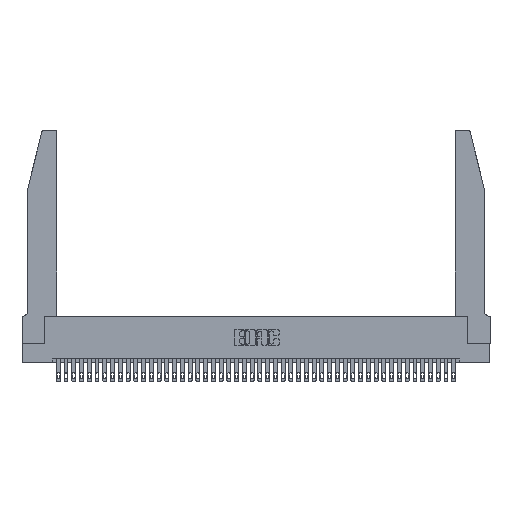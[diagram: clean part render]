
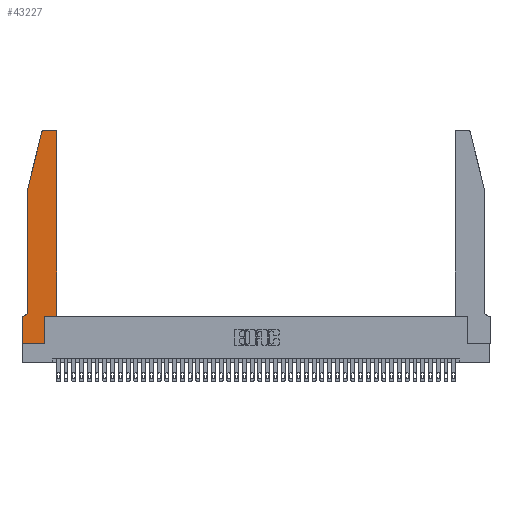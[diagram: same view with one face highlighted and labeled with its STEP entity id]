
A CAD part, top view. The second image highlights one B-rep face of the part: STEP entity #43227.
In plain terms, the highlighted planar face has unit normal (0, 0, 1).
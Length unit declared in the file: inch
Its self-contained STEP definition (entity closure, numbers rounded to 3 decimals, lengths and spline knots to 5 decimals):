
#622 = DIRECTION ( 'NONE',  ( 1., 0., 0. ) ) ;
#659 = CARTESIAN_POINT ( 'NONE',  ( 0.0755, 2., 0.37 ) ) ;
#669 = VECTOR ( 'NONE', #16665, 39.37008 ) ;
#737 = EDGE_CURVE ( 'NONE', #5990, #23715, #5614, .T. ) ;
#746 = CARTESIAN_POINT ( 'NONE',  ( 0., 0., 0.37 ) ) ;
#941 = ORIENTED_EDGE ( 'NONE', *, *, #5245, .T. ) ;
#997 = AXIS2_PLACEMENT_3D ( 'NONE', #36835, #16348, #6878 ) ;
#1511 = VECTOR ( 'NONE', #34102, 39.37008 ) ;
#1585 = CARTESIAN_POINT ( 'NONE',  ( 0.0755, 2., 0.37 ) ) ;
#1917 = CARTESIAN_POINT ( 'NONE',  ( 0.4205, 2.72, 0.37 ) ) ;
#2085 = ORIENTED_EDGE ( 'NONE', *, *, #23469, .T. ) ;
#2121 = CARTESIAN_POINT ( 'NONE',  ( 0.0055, 0.35, 0.37 ) ) ;
#2169 = CARTESIAN_POINT ( 'NONE',  ( 0.0755, 0.42, 0.37 ) ) ;
#2500 = VERTEX_POINT ( 'NONE', #10021 ) ;
#2548 = VECTOR ( 'NONE', #10915, 39.37008 ) ;
#2983 = ORIENTED_EDGE ( 'NONE', *, *, #7462, .T. ) ;
#3103 = LINE ( 'NONE', #7789, #33098 ) ;
#4253 = VERTEX_POINT ( 'NONE', #24891 ) ;
#4413 = VERTEX_POINT ( 'NONE', #15961 ) ;
#5015 = ORIENTED_EDGE ( 'NONE', *, *, #9977, .T. ) ;
#5245 = EDGE_CURVE ( 'NONE', #37400, #27369, #27476, .T. ) ;
#5614 = LINE ( 'NONE', #23602, #23258 ) ;
#5781 = VECTOR ( 'NONE', #25886, 39.37008 ) ;
#5990 = VERTEX_POINT ( 'NONE', #17314 ) ;
#6348 = DIRECTION ( 'NONE',  ( 0., -1., 0. ) ) ;
#6668 = EDGE_CURVE ( 'NONE', #4413, #11718, #29048, .T. ) ;
#6878 = DIRECTION ( 'NONE',  ( 1., 0., 0. ) ) ;
#6927 = EDGE_CURVE ( 'NONE', #13416, #5990, #22099, .T. ) ;
#7017 = LINE ( 'NONE', #14941, #35959 ) ;
#7110 = VECTOR ( 'NONE', #24988, 39.37008 ) ;
#7462 = EDGE_CURVE ( 'NONE', #28771, #40537, #7017, .T. ) ;
#7734 = ORIENTED_EDGE ( 'NONE', *, *, #6668, .T. ) ;
#7789 = CARTESIAN_POINT ( 'NONE',  ( 0.2605, 2.75, 0.37 ) ) ;
#9977 = EDGE_CURVE ( 'NONE', #16916, #4253, #10540, .T. ) ;
#10021 = CARTESIAN_POINT ( 'NONE',  ( 0.4205, 2.75, 0.37 ) ) ;
#10369 = AXIS2_PLACEMENT_3D ( 'NONE', #1917, #18962, #26243 ) ;
#10540 = LINE ( 'NONE', #43787, #1511 ) ;
#10915 = DIRECTION ( 'NONE',  ( 0., 1., 0. ) ) ;
#11714 = EDGE_CURVE ( 'NONE', #40537, #13416, #22880, .T. ) ;
#11718 = VERTEX_POINT ( 'NONE', #38920 ) ;
#11804 = FACE_OUTER_BOUND ( 'NONE', #36559, .T. ) ;
#13416 = VERTEX_POINT ( 'NONE', #34346 ) ;
#13511 = EDGE_CURVE ( 'NONE', #4253, #28771, #16256, .T. ) ;
#14941 = CARTESIAN_POINT ( 'NONE',  ( 0., 0., 0.37 ) ) ;
#14964 = CARTESIAN_POINT ( 'NONE',  ( 0.2865, 0., 0.37 ) ) ;
#15961 = CARTESIAN_POINT ( 'NONE',  ( 0.284, 2.75, 0.37 ) ) ;
#16256 = LINE ( 'NONE', #30144, #18978 ) ;
#16348 = DIRECTION ( 'NONE',  ( 0., 0., 1. ) ) ;
#16665 = DIRECTION ( 'NONE',  ( 1., 0., 0. ) ) ;
#16750 = EDGE_CURVE ( 'NONE', #2500, #4413, #3103, .T. ) ;
#16828 = EDGE_CURVE ( 'NONE', #11718, #37400, #40034, .T. ) ;
#16916 = VERTEX_POINT ( 'NONE', #2121 ) ;
#17314 = CARTESIAN_POINT ( 'NONE',  ( 0.4505, 0.35, 0.37 ) ) ;
#18962 = DIRECTION ( 'NONE',  ( 0., 0., 1. ) ) ;
#18978 = VECTOR ( 'NONE', #6348, 39.37008 ) ;
#19290 = ORIENTED_EDGE ( 'NONE', *, *, #16750, .T. ) ;
#21100 = ORIENTED_EDGE ( 'NONE', *, *, #13511, .T. ) ;
#21734 = CARTESIAN_POINT ( 'NONE',  ( 0.0755, 2., 0.37 ) ) ;
#22099 = LINE ( 'NONE', #26092, #669 ) ;
#22880 = LINE ( 'NONE', #43933, #2548 ) ;
#23258 = VECTOR ( 'NONE', #37070, 39.37008 ) ;
#23361 = ORIENTED_EDGE ( 'NONE', *, *, #11714, .T. ) ;
#23469 = EDGE_CURVE ( 'NONE', #27369, #16916, #39064, .T. ) ;
#23602 = CARTESIAN_POINT ( 'NONE',  ( 0.4505, 0.35, 0.37 ) ) ;
#23715 = VERTEX_POINT ( 'NONE', #25215 ) ;
#24795 = ORIENTED_EDGE ( 'NONE', *, *, #16828, .T. ) ;
#24891 = CARTESIAN_POINT ( 'NONE',  ( 0., 0.35, 0.37 ) ) ;
#24988 = DIRECTION ( 'NONE',  ( 0., -1., 0. ) ) ;
#25031 = AXIS2_PLACEMENT_3D ( 'NONE', #41374, #30810, #622 ) ;
#25215 = CARTESIAN_POINT ( 'NONE',  ( 0.4505, 2.72, 0.37 ) ) ;
#25886 = DIRECTION ( 'NONE',  ( -0.239, -0.971, 0. ) ) ;
#26092 = CARTESIAN_POINT ( 'NONE',  ( 0.4505, 0.35, 0.37 ) ) ;
#26243 = DIRECTION ( 'NONE',  ( 1., 0., 0. ) ) ;
#26548 = DIRECTION ( 'NONE',  ( -1., 0., 0. ) ) ;
#27369 = VERTEX_POINT ( 'NONE', #2169 ) ;
#27476 = LINE ( 'NONE', #21734, #7110 ) ;
#28443 = DIRECTION ( 'NONE',  ( -1., 0., 0. ) ) ;
#28679 = ORIENTED_EDGE ( 'NONE', *, *, #41401, .T. ) ;
#28771 = VERTEX_POINT ( 'NONE', #746 ) ;
#29048 = CIRCLE ( 'NONE', #997, 0.03 ) ;
#30144 = CARTESIAN_POINT ( 'NONE',  ( 0., 0., 0.37 ) ) ;
#30810 = DIRECTION ( 'NONE',  ( 0., 0., 1. ) ) ;
#31519 = AXIS2_PLACEMENT_3D ( 'NONE', #33029, #33458, #26548 ) ;
#33029 = CARTESIAN_POINT ( 'NONE',  ( 0.0055, 0.42, 0.37 ) ) ;
#33098 = VECTOR ( 'NONE', #28443, 39.37008 ) ;
#33458 = DIRECTION ( 'NONE',  ( 0., 0., -1. ) ) ;
#34102 = DIRECTION ( 'NONE',  ( -1., 0., 0. ) ) ;
#34346 = CARTESIAN_POINT ( 'NONE',  ( 0.2865, 0.35, 0.37 ) ) ;
#35883 = DIRECTION ( 'NONE',  ( 1., 0., 0. ) ) ;
#35959 = VECTOR ( 'NONE', #35883, 39.37008 ) ;
#36559 = EDGE_LOOP ( 'NONE', ( #19290, #7734, #24795, #941, #2085, #5015, #21100, #2983, #23361, #38832, #38585, #28679 ) ) ;
#36835 = CARTESIAN_POINT ( 'NONE',  ( 0.284, 2.72, 0.37 ) ) ;
#37070 = DIRECTION ( 'NONE',  ( 0., 1., 0. ) ) ;
#37400 = VERTEX_POINT ( 'NONE', #659 ) ;
#38585 = ORIENTED_EDGE ( 'NONE', *, *, #737, .T. ) ;
#38832 = ORIENTED_EDGE ( 'NONE', *, *, #6927, .T. ) ;
#38920 = CARTESIAN_POINT ( 'NONE',  ( 0.25487, 2.72718, 0.37 ) ) ;
#39064 = CIRCLE ( 'NONE', #31519, 0.07 ) ;
#40034 = LINE ( 'NONE', #1585, #5781 ) ;
#40537 = VERTEX_POINT ( 'NONE', #14964 ) ;
#41239 = PLANE ( 'NONE',  #25031 ) ;
#41374 = CARTESIAN_POINT ( 'NONE',  ( 0., 0.35, 0.37 ) ) ;
#41401 = EDGE_CURVE ( 'NONE', #23715, #2500, #43503, .T. ) ;
#43227 = ADVANCED_FACE ( 'NONE', ( #11804 ), #41239, .T. ) ;
#43503 = CIRCLE ( 'NONE', #10369, 0.03 ) ;
#43787 = CARTESIAN_POINT ( 'NONE',  ( 0.0755, 0.35, 0.37 ) ) ;
#43933 = CARTESIAN_POINT ( 'NONE',  ( 0.2865, 0.35, 0.37 ) ) ;
